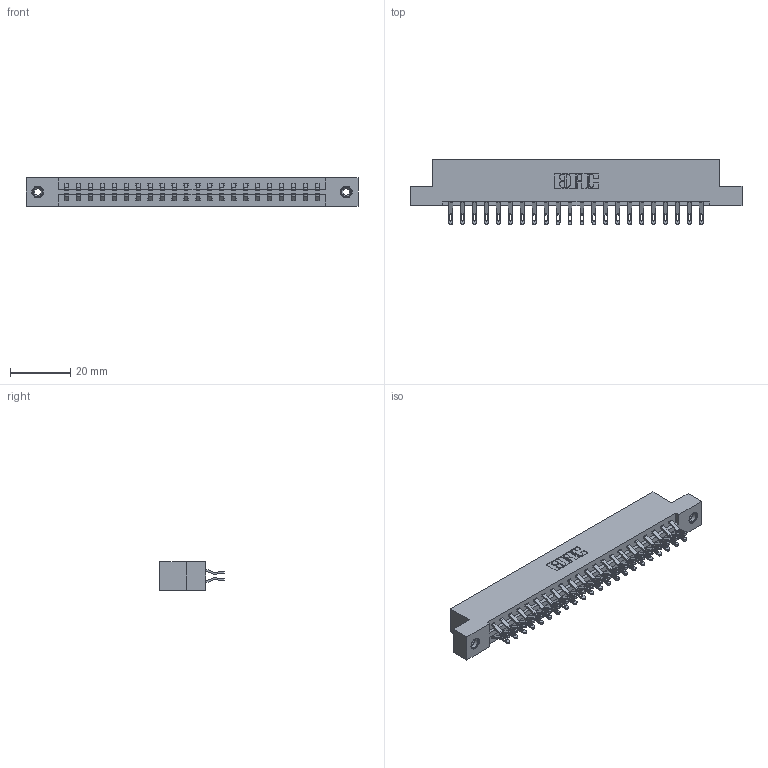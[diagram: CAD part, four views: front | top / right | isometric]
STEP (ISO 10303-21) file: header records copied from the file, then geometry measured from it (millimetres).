
FILE_DESCRIPTION (( 'STEP AP203' ), '1' );
FILE_NAME ('387-044-555-208.STEP', '2018-09-20T02:37:54', ( '' ), ( '' ), 'SwSTEP 2.0', 'SolidWorks 2016', '' );
FILE_SCHEMA (( 'CONFIG_CONTROL_DESIGN' ));
Length unit declared in the file: inch
Products named in the file (4): 345-292-001_555 Tail; 345-250-001_345-250-003-102; 387-044-555-208; 337 Part_Flush Mounting Lugs - 0.156 Dia-TI
Assembly tree (47 placements, depth 2):
  387-044-555-208
    337 Part_Flush Mounting Lugs - 0.156 Dia-TI
    345-292-001_555 Tail  x44
    345-250-001_345-250-003-102  x2
Bounding box: 110.19 x 21.47 x 9.4 mm (x, y, z)
Volume: 11467.1 mm3; surface area: 13274.2 mm2
Topology: 47 solids, 47 shells, 2814 faces, 8763 edges, 5834 vertices
Faces by surface type: plane 1686, cylinder 1112, cone 12, torus 4
Entity records: 21156 total; most frequent: CARTESIAN_POINT 3595, ORIENTED_EDGE 3494, DIRECTION 3097, EDGE_CURVE 1747, LINE 1579, VECTOR 1579, VERTEX_POINT 1160, AXIS2_PLACEMENT_3D 759
